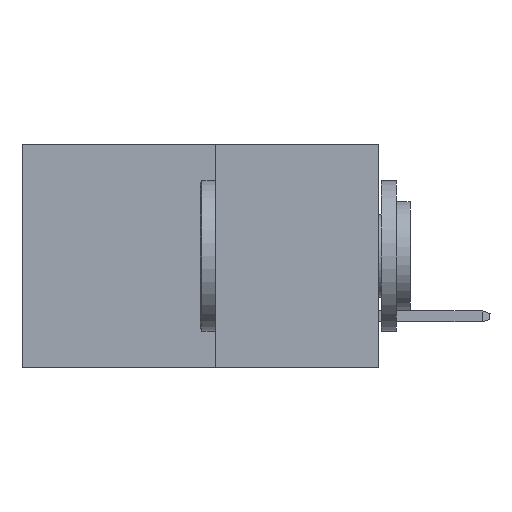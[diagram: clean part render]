
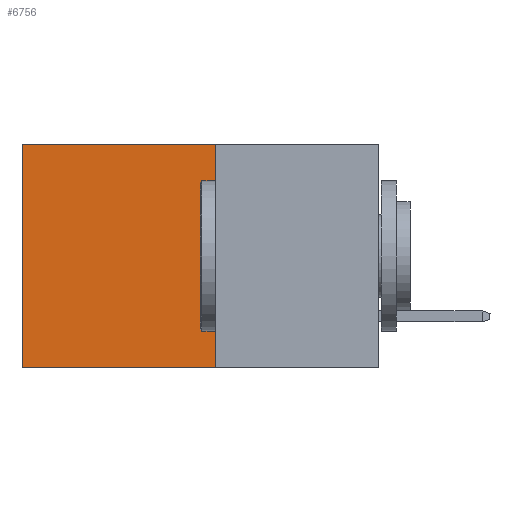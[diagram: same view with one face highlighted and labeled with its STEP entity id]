
A CAD part, left-side view. The second image highlights one B-rep face of the part: STEP entity #6756.
In plain terms, the highlighted planar face has unit normal (-1, 0, 0).
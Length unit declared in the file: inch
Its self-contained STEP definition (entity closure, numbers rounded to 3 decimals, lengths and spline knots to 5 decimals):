
#742 = LINE ( 'NONE', #13995, #9512 ) ;
#1026 = ORIENTED_EDGE ( 'NONE', *, *, #11421, .F. ) ;
#1666 = DIRECTION ( 'NONE',  ( 0., 1., 0. ) ) ;
#2222 = LINE ( 'NONE', #13868, #5649 ) ;
#2667 = DIRECTION ( 'NONE',  ( 0., 1., 0. ) ) ;
#2894 = VERTEX_POINT ( 'NONE', #9209 ) ;
#3897 = DIRECTION ( 'NONE',  ( 0., 0., -1. ) ) ;
#4492 = ORIENTED_EDGE ( 'NONE', *, *, #12053, .T. ) ;
#4810 = EDGE_CURVE ( 'NONE', #6794, #11573, #6141, .T. ) ;
#5649 = VECTOR ( 'NONE', #3897, 39.37008 ) ;
#6141 = LINE ( 'NONE', #10620, #9124 ) ;
#6497 = CARTESIAN_POINT ( 'NONE',  ( 0.277, 0.59, -0.37 ) ) ;
#6756 = ADVANCED_FACE ( 'NONE', ( #12851 ), #12700, .F. ) ;
#6794 = VERTEX_POINT ( 'NONE', #6875 ) ;
#6875 = CARTESIAN_POINT ( 'NONE',  ( 0.277, 0.59, 0. ) ) ;
#7219 = CARTESIAN_POINT ( 'NONE',  ( 0.277, 0.27, 0. ) ) ;
#8142 = AXIS2_PLACEMENT_3D ( 'NONE', #13460, #14519, #14193 ) ;
#9124 = VECTOR ( 'NONE', #10867, 39.37008 ) ;
#9209 = CARTESIAN_POINT ( 'NONE',  ( 0.277, 0.27, 0. ) ) ;
#9342 = EDGE_CURVE ( 'NONE', #2894, #13874, #2222, .T. ) ;
#9512 = VECTOR ( 'NONE', #1666, 39.37008 ) ;
#9940 = EDGE_LOOP ( 'NONE', ( #12723, #1026, #13044, #4492 ) ) ;
#10010 = VECTOR ( 'NONE', #2667, 39.37008 ) ;
#10354 = LINE ( 'NONE', #7219, #10010 ) ;
#10620 = CARTESIAN_POINT ( 'NONE',  ( 0.277, 0.59, -0.37 ) ) ;
#10867 = DIRECTION ( 'NONE',  ( 0., 0., -1. ) ) ;
#11421 = EDGE_CURVE ( 'NONE', #13874, #11573, #742, .T. ) ;
#11573 = VERTEX_POINT ( 'NONE', #6497 ) ;
#11910 = CARTESIAN_POINT ( 'NONE',  ( 0.277, 0.27, -0.37 ) ) ;
#12053 = EDGE_CURVE ( 'NONE', #2894, #6794, #10354, .T. ) ;
#12700 = PLANE ( 'NONE',  #8142 ) ;
#12723 = ORIENTED_EDGE ( 'NONE', *, *, #4810, .T. ) ;
#12851 = FACE_OUTER_BOUND ( 'NONE', #9940, .T. ) ;
#13044 = ORIENTED_EDGE ( 'NONE', *, *, #9342, .F. ) ;
#13460 = CARTESIAN_POINT ( 'NONE',  ( 0.277, 0.27, -0.37 ) ) ;
#13868 = CARTESIAN_POINT ( 'NONE',  ( 0.277, 0.27, -0.37 ) ) ;
#13874 = VERTEX_POINT ( 'NONE', #11910 ) ;
#13995 = CARTESIAN_POINT ( 'NONE',  ( 0.277, 0.27, -0.37 ) ) ;
#14193 = DIRECTION ( 'NONE',  ( 0., 0., -1. ) ) ;
#14519 = DIRECTION ( 'NONE',  ( 1., 0., 0. ) ) ;
